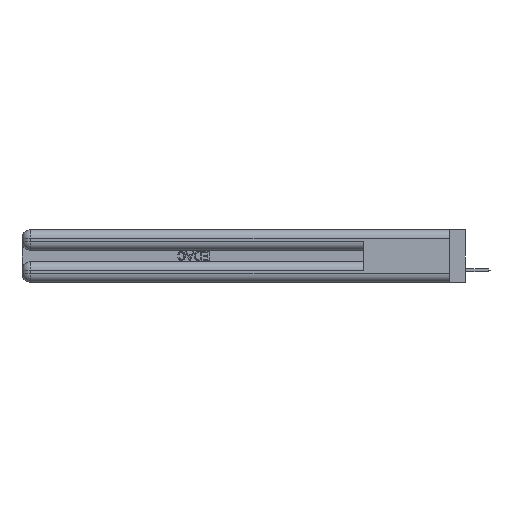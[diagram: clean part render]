
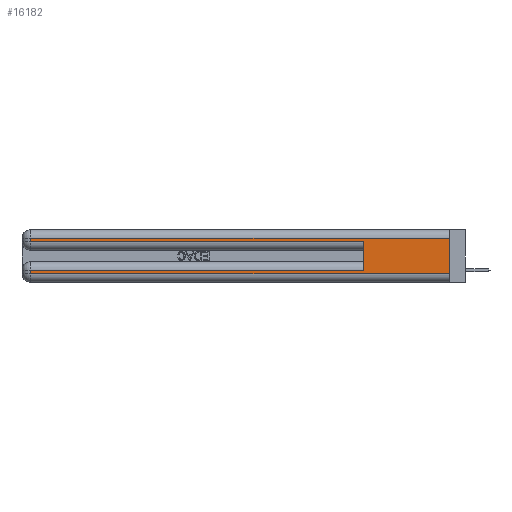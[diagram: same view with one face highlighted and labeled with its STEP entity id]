
A CAD part, left-side view. The second image highlights one B-rep face of the part: STEP entity #16182.
In plain terms, the highlighted planar face has unit normal (-1, 0, 0).
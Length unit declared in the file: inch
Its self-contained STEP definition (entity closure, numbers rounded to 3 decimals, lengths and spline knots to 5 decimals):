
#864 = VECTOR ( 'NONE', #45070, 39.37008 ) ;
#2429 = ORIENTED_EDGE ( 'NONE', *, *, #14604, .F. ) ;
#2447 = AXIS2_PLACEMENT_3D ( 'NONE', #41172, #30619, #8997 ) ;
#2558 = ORIENTED_EDGE ( 'NONE', *, *, #38134, .T. ) ;
#2905 = LINE ( 'NONE', #25565, #24228 ) ;
#3331 = CARTESIAN_POINT ( 'NONE',  ( 0., 2.94, 0.06 ) ) ;
#3754 = DIRECTION ( 'NONE',  ( 0., 1., 0. ) ) ;
#3919 = LINE ( 'NONE', #5063, #15736 ) ;
#5063 = CARTESIAN_POINT ( 'NONE',  ( 0., 0., 0.37 ) ) ;
#5292 = VERTEX_POINT ( 'NONE', #25947 ) ;
#5629 = VERTEX_POINT ( 'NONE', #34931 ) ;
#5631 = VERTEX_POINT ( 'NONE', #3331 ) ;
#5635 = DIRECTION ( 'NONE',  ( 0., -1., 0. ) ) ;
#6127 = CARTESIAN_POINT ( 'NONE',  ( 0., 2.94, 0.085 ) ) ;
#7841 = VECTOR ( 'NONE', #5635, 39.37008 ) ;
#8508 = EDGE_LOOP ( 'NONE', ( #2429, #31701, #2558, #44379, #35431, #43468, #39412, #22971 ) ) ;
#8962 = CARTESIAN_POINT ( 'NONE',  ( 0., 0.6, 0.285 ) ) ;
#8981 = LINE ( 'NONE', #37872, #7841 ) ;
#8997 = DIRECTION ( 'NONE',  ( 0., 0., -1. ) ) ;
#9070 = VERTEX_POINT ( 'NONE', #8962 ) ;
#9268 = VECTOR ( 'NONE', #40822, 39.37008 ) ;
#10252 = CARTESIAN_POINT ( 'NONE',  ( 0., 0.6, 0.145 ) ) ;
#10482 = LINE ( 'NONE', #39316, #30070 ) ;
#10782 = DIRECTION ( 'NONE',  ( 0., 0., -1. ) ) ;
#11889 = EDGE_CURVE ( 'NONE', #23014, #5631, #10482, .T. ) ;
#12363 = EDGE_CURVE ( 'NONE', #22128, #23014, #26147, .T. ) ;
#12825 = CARTESIAN_POINT ( 'NONE',  ( 0., 0., 0.31 ) ) ;
#14604 = EDGE_CURVE ( 'NONE', #33786, #5629, #3919, .T. ) ;
#15736 = VECTOR ( 'NONE', #19564, 39.37008 ) ;
#16061 = VECTOR ( 'NONE', #45425, 39.37008 ) ;
#16182 = ADVANCED_FACE ( 'NONE', ( #26779 ), #26897, .F. ) ;
#19564 = DIRECTION ( 'NONE',  ( 0., 0., -1. ) ) ;
#19820 = CARTESIAN_POINT ( 'NONE',  ( 0., 2.94, 0.285 ) ) ;
#20281 = CARTESIAN_POINT ( 'NONE',  ( 0., 2.94, 0.37 ) ) ;
#22128 = VERTEX_POINT ( 'NONE', #36382 ) ;
#22148 = LINE ( 'NONE', #20281, #864 ) ;
#22971 = ORIENTED_EDGE ( 'NONE', *, *, #24863, .T. ) ;
#23014 = VERTEX_POINT ( 'NONE', #6127 ) ;
#24228 = VECTOR ( 'NONE', #3754, 39.37008 ) ;
#24863 = EDGE_CURVE ( 'NONE', #5631, #5629, #8981, .T. ) ;
#25565 = CARTESIAN_POINT ( 'NONE',  ( 0., 0., 0.31 ) ) ;
#25947 = CARTESIAN_POINT ( 'NONE',  ( 0., 2.94, 0.31 ) ) ;
#26147 = LINE ( 'NONE', #34511, #16061 ) ;
#26779 = FACE_OUTER_BOUND ( 'NONE', #8508, .T. ) ;
#26897 = PLANE ( 'NONE',  #2447 ) ;
#29467 = LINE ( 'NONE', #37264, #9268 ) ;
#29983 = EDGE_CURVE ( 'NONE', #43114, #9070, #29467, .T. ) ;
#30070 = VECTOR ( 'NONE', #10782, 39.37008 ) ;
#30619 = DIRECTION ( 'NONE',  ( 1., 0., 0. ) ) ;
#31701 = ORIENTED_EDGE ( 'NONE', *, *, #32965, .T. ) ;
#31749 = EDGE_CURVE ( 'NONE', #22128, #9070, #36052, .T. ) ;
#32965 = EDGE_CURVE ( 'NONE', #33786, #5292, #2905, .T. ) ;
#33786 = VERTEX_POINT ( 'NONE', #12825 ) ;
#34511 = CARTESIAN_POINT ( 'NONE',  ( 0., 0., 0.085 ) ) ;
#34931 = CARTESIAN_POINT ( 'NONE',  ( 0., 0., 0.06 ) ) ;
#35431 = ORIENTED_EDGE ( 'NONE', *, *, #31749, .F. ) ;
#36052 = LINE ( 'NONE', #10252, #42205 ) ;
#36382 = CARTESIAN_POINT ( 'NONE',  ( 0., 0.6, 0.085 ) ) ;
#37264 = CARTESIAN_POINT ( 'NONE',  ( 0., 0., 0.285 ) ) ;
#37872 = CARTESIAN_POINT ( 'NONE',  ( 0., 0., 0.06 ) ) ;
#38134 = EDGE_CURVE ( 'NONE', #5292, #43114, #22148, .T. ) ;
#38174 = DIRECTION ( 'NONE',  ( 0., 0., 1. ) ) ;
#39316 = CARTESIAN_POINT ( 'NONE',  ( 0., 2.94, 0.37 ) ) ;
#39412 = ORIENTED_EDGE ( 'NONE', *, *, #11889, .T. ) ;
#40822 = DIRECTION ( 'NONE',  ( 0., -1., 0. ) ) ;
#41172 = CARTESIAN_POINT ( 'NONE',  ( 0., 0., 0.37 ) ) ;
#42205 = VECTOR ( 'NONE', #38174, 39.37008 ) ;
#43114 = VERTEX_POINT ( 'NONE', #19820 ) ;
#43468 = ORIENTED_EDGE ( 'NONE', *, *, #12363, .T. ) ;
#44379 = ORIENTED_EDGE ( 'NONE', *, *, #29983, .T. ) ;
#45070 = DIRECTION ( 'NONE',  ( 0., 0., -1. ) ) ;
#45425 = DIRECTION ( 'NONE',  ( 0., 1., 0. ) ) ;
